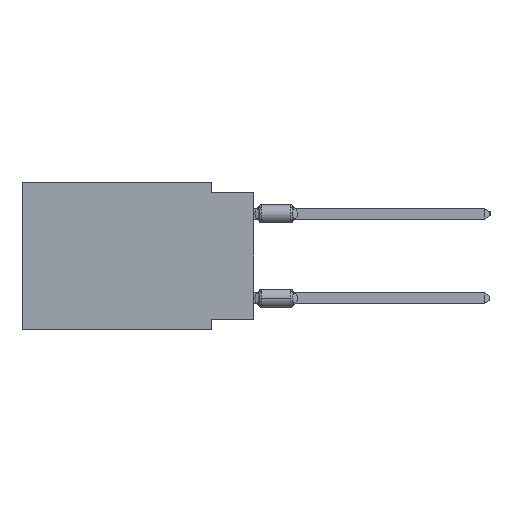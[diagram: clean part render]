
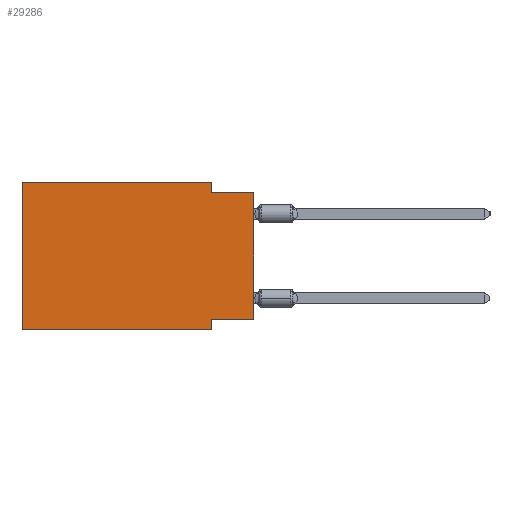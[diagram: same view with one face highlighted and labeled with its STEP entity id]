
A CAD part, left-side view. The second image highlights one B-rep face of the part: STEP entity #29286.
In plain terms, the highlighted planar face has unit normal (-1, 0, 0).
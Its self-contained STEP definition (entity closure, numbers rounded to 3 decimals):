
#262 = VERTEX_POINT ( 'NONE', #38432 ) ;
#553 = PLANE ( 'NONE',  #16695 ) ;
#597 = CARTESIAN_POINT ( 'NONE',  ( 0., 0., -8.255 ) ) ;
#1255 = CARTESIAN_POINT ( 'NONE',  ( 0., 0., -0.635 ) ) ;
#2030 = VERTEX_POINT ( 'NONE', #597 ) ;
#3186 = CARTESIAN_POINT ( 'NONE',  ( 0., 2.54, -8.89 ) ) ;
#3483 = DIRECTION ( 'NONE',  ( 0., 0., -1. ) ) ;
#3858 = CARTESIAN_POINT ( 'NONE',  ( 0., 2.54, 0. ) ) ;
#5189 = FACE_OUTER_BOUND ( 'NONE', #34203, .T. ) ;
#5808 = ORIENTED_EDGE ( 'NONE', *, *, #52392, .F. ) ;
#6633 = CARTESIAN_POINT ( 'NONE',  ( 0., 2.54, -8.255 ) ) ;
#7328 = VECTOR ( 'NONE', #18239, 1000. ) ;
#7493 = LINE ( 'NONE', #3186, #29907 ) ;
#8994 = CARTESIAN_POINT ( 'NONE',  ( 0., 13.97, 0. ) ) ;
#10533 = LINE ( 'NONE', #15463, #40583 ) ;
#11032 = CARTESIAN_POINT ( 'NONE',  ( 0., 13.97, 0. ) ) ;
#12067 = EDGE_CURVE ( 'NONE', #2030, #47313, #46559, .T. ) ;
#12808 = LINE ( 'NONE', #3858, #36851 ) ;
#14307 = VECTOR ( 'NONE', #23981, 1000. ) ;
#14823 = LINE ( 'NONE', #1255, #44121 ) ;
#15463 = CARTESIAN_POINT ( 'NONE',  ( 0., 13.97, -8.89 ) ) ;
#15908 = EDGE_CURVE ( 'NONE', #47313, #46600, #7493, .T. ) ;
#16695 = AXIS2_PLACEMENT_3D ( 'NONE', #11032, #24311, #57029 ) ;
#18188 = EDGE_CURVE ( 'NONE', #262, #27890, #12808, .T. ) ;
#18239 = DIRECTION ( 'NONE',  ( 0., 0., 1. ) ) ;
#18768 = VECTOR ( 'NONE', #20435, 1000. ) ;
#19605 = ORIENTED_EDGE ( 'NONE', *, *, #25330, .F. ) ;
#20056 = DIRECTION ( 'NONE',  ( 0., -1., 0. ) ) ;
#20435 = DIRECTION ( 'NONE',  ( 0., 0., 1. ) ) ;
#21754 = ORIENTED_EDGE ( 'NONE', *, *, #54909, .F. ) ;
#23981 = DIRECTION ( 'NONE',  ( 0., 1., 0. ) ) ;
#24311 = DIRECTION ( 'NONE',  ( 1., 0., 0. ) ) ;
#25330 = EDGE_CURVE ( 'NONE', #51583, #31488, #42320, .T. ) ;
#27668 = CARTESIAN_POINT ( 'NONE',  ( 0., 13.97, 0. ) ) ;
#27890 = VERTEX_POINT ( 'NONE', #50853 ) ;
#28009 = CARTESIAN_POINT ( 'NONE',  ( 0., 0., -0.635 ) ) ;
#28104 = CARTESIAN_POINT ( 'NONE',  ( 0., 13.97, 0. ) ) ;
#29286 = ADVANCED_FACE ( 'NONE', ( #5189 ), #553, .F. ) ;
#29708 = ORIENTED_EDGE ( 'NONE', *, *, #18188, .F. ) ;
#29907 = VECTOR ( 'NONE', #3483, 1000. ) ;
#31488 = VERTEX_POINT ( 'NONE', #28104 ) ;
#32458 = CARTESIAN_POINT ( 'NONE',  ( 0., 2.54, -8.89 ) ) ;
#33139 = ORIENTED_EDGE ( 'NONE', *, *, #38058, .T. ) ;
#34203 = EDGE_LOOP ( 'NONE', ( #36538, #5808, #29708, #21754, #19605, #33139, #56197, #46858 ) ) ;
#34313 = DIRECTION ( 'NONE',  ( 0., -1., 0. ) ) ;
#34657 = LINE ( 'NONE', #34961, #18768 ) ;
#34961 = CARTESIAN_POINT ( 'NONE',  ( 0., 0., 0. ) ) ;
#36538 = ORIENTED_EDGE ( 'NONE', *, *, #44934, .T. ) ;
#36851 = VECTOR ( 'NONE', #41521, 1000. ) ;
#37088 = VECTOR ( 'NONE', #42151, 1000. ) ;
#38058 = EDGE_CURVE ( 'NONE', #51583, #46600, #10533, .T. ) ;
#38432 = CARTESIAN_POINT ( 'NONE',  ( 0., 2.54, 0. ) ) ;
#40583 = VECTOR ( 'NONE', #34313, 1000. ) ;
#41521 = DIRECTION ( 'NONE',  ( 0., 0., -1. ) ) ;
#42151 = DIRECTION ( 'NONE',  ( 0., -1., 0. ) ) ;
#42320 = LINE ( 'NONE', #8994, #7328 ) ;
#44121 = VECTOR ( 'NONE', #20056, 1000. ) ;
#44934 = EDGE_CURVE ( 'NONE', #2030, #58139, #34657, .T. ) ;
#45600 = LINE ( 'NONE', #27668, #37088 ) ;
#46559 = LINE ( 'NONE', #56407, #14307 ) ;
#46600 = VERTEX_POINT ( 'NONE', #32458 ) ;
#46858 = ORIENTED_EDGE ( 'NONE', *, *, #12067, .F. ) ;
#47313 = VERTEX_POINT ( 'NONE', #6633 ) ;
#50853 = CARTESIAN_POINT ( 'NONE',  ( 0., 2.54, -0.635 ) ) ;
#51583 = VERTEX_POINT ( 'NONE', #53546 ) ;
#52392 = EDGE_CURVE ( 'NONE', #27890, #58139, #14823, .T. ) ;
#53546 = CARTESIAN_POINT ( 'NONE',  ( 0., 13.97, -8.89 ) ) ;
#54909 = EDGE_CURVE ( 'NONE', #31488, #262, #45600, .T. ) ;
#56197 = ORIENTED_EDGE ( 'NONE', *, *, #15908, .F. ) ;
#56407 = CARTESIAN_POINT ( 'NONE',  ( 0., 0., -8.255 ) ) ;
#57029 = DIRECTION ( 'NONE',  ( 0., 0., -1. ) ) ;
#58139 = VERTEX_POINT ( 'NONE', #28009 ) ;
